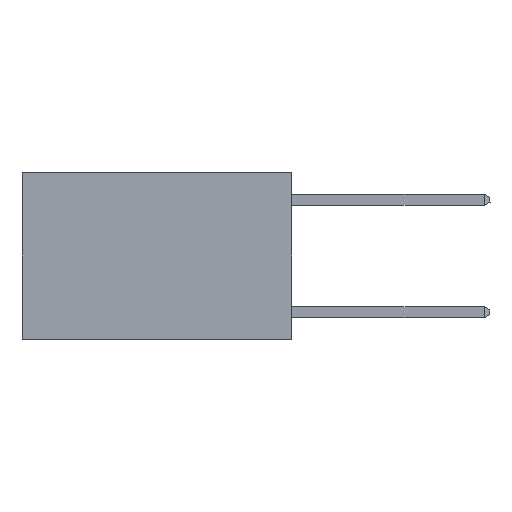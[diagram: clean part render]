
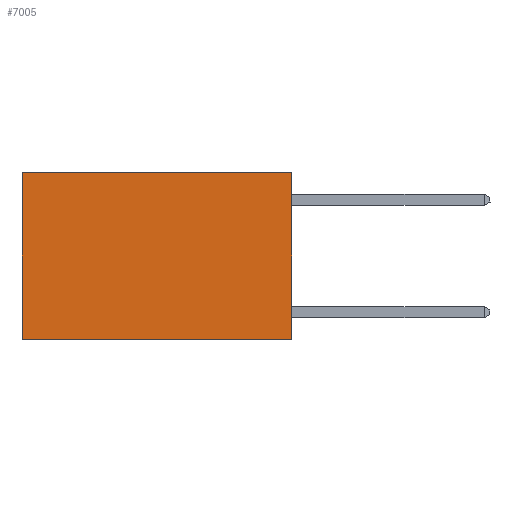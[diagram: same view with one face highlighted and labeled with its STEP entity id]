
A CAD part, left-side view. The second image highlights one B-rep face of the part: STEP entity #7005.
In plain terms, the highlighted planar face has unit normal (-1, 0, 0).
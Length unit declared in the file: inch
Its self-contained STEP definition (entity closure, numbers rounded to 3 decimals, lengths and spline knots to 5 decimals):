
#49 = DIRECTION ( 'NONE',  ( 0., 1., 0. ) ) ;
#58 = CARTESIAN_POINT ( 'NONE',  ( 0.2625, 0., 0. ) ) ;
#361 = EDGE_CURVE ( 'NONE', #6711, #8154, #984, .T. ) ;
#694 = DIRECTION ( 'NONE',  ( 0., 0., -1. ) ) ;
#759 = DIRECTION ( 'NONE',  ( 1., 0., 0. ) ) ;
#984 = LINE ( 'NONE', #4591, #2591 ) ;
#1170 = DIRECTION ( 'NONE',  ( 0., 0., -1. ) ) ;
#1477 = ORIENTED_EDGE ( 'NONE', *, *, #4708, .T. ) ;
#1676 = ORIENTED_EDGE ( 'NONE', *, *, #5407, .F. ) ;
#1754 = ORIENTED_EDGE ( 'NONE', *, *, #7277, .F. ) ;
#2234 = ORIENTED_EDGE ( 'NONE', *, *, #361, .T. ) ;
#2485 = VECTOR ( 'NONE', #1170, 39.37008 ) ;
#2591 = VECTOR ( 'NONE', #49, 39.37008 ) ;
#3901 = EDGE_LOOP ( 'NONE', ( #1477, #1676, #1754, #2234 ) ) ;
#4139 = PLANE ( 'NONE',  #7013 ) ;
#4394 = VERTEX_POINT ( 'NONE', #6351 ) ;
#4591 = CARTESIAN_POINT ( 'NONE',  ( 0.2625, 0., 0. ) ) ;
#4708 = EDGE_CURVE ( 'NONE', #8154, #4394, #5041, .T. ) ;
#4727 = VERTEX_POINT ( 'NONE', #7952 ) ;
#4842 = VECTOR ( 'NONE', #694, 39.37008 ) ;
#4845 = DIRECTION ( 'NONE',  ( 0., 1., 0. ) ) ;
#4929 = VECTOR ( 'NONE', #4845, 39.37008 ) ;
#5041 = LINE ( 'NONE', #7320, #4842 ) ;
#5175 = CARTESIAN_POINT ( 'NONE',  ( 0.2625, 0., 0. ) ) ;
#5407 = EDGE_CURVE ( 'NONE', #4727, #4394, #6442, .T. ) ;
#5412 = CARTESIAN_POINT ( 'NONE',  ( 0.2625, 0.6, 0. ) ) ;
#5451 = DIRECTION ( 'NONE',  ( 0., 0., -1. ) ) ;
#5492 = CARTESIAN_POINT ( 'NONE',  ( 0.2625, 0., -0.37 ) ) ;
#6013 = LINE ( 'NONE', #7123, #2485 ) ;
#6351 = CARTESIAN_POINT ( 'NONE',  ( 0.2625, 0.6, -0.37 ) ) ;
#6442 = LINE ( 'NONE', #5492, #4929 ) ;
#6711 = VERTEX_POINT ( 'NONE', #5175 ) ;
#7005 = ADVANCED_FACE ( 'NONE', ( #8181 ), #4139, .F. ) ;
#7013 = AXIS2_PLACEMENT_3D ( 'NONE', #58, #759, #5451 ) ;
#7123 = CARTESIAN_POINT ( 'NONE',  ( 0.2625, 0., 0. ) ) ;
#7277 = EDGE_CURVE ( 'NONE', #6711, #4727, #6013, .T. ) ;
#7320 = CARTESIAN_POINT ( 'NONE',  ( 0.2625, 0.6, 0. ) ) ;
#7952 = CARTESIAN_POINT ( 'NONE',  ( 0.2625, 0., -0.37 ) ) ;
#8154 = VERTEX_POINT ( 'NONE', #5412 ) ;
#8181 = FACE_OUTER_BOUND ( 'NONE', #3901, .T. ) ;
